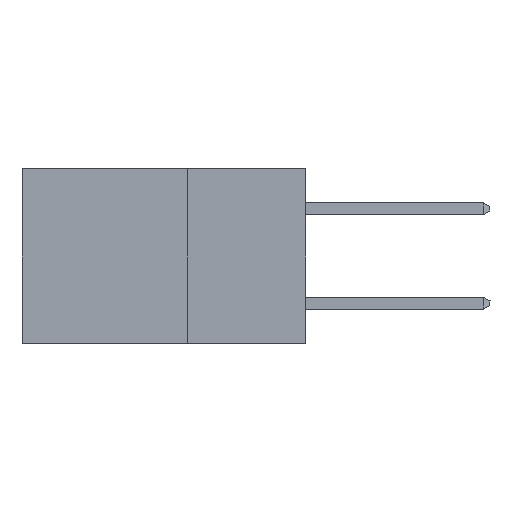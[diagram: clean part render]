
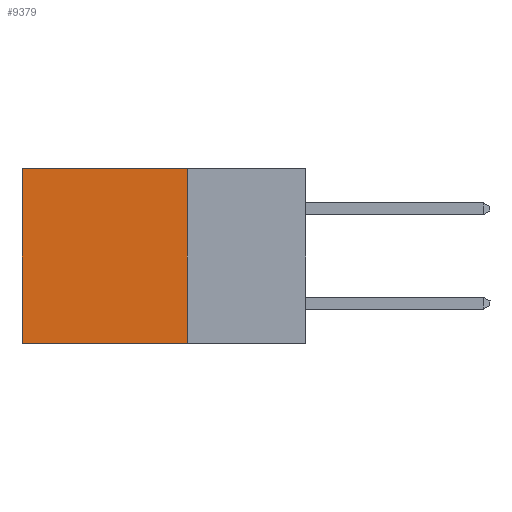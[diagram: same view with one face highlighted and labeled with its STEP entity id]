
A CAD part, left-side view. The second image highlights one B-rep face of the part: STEP entity #9379.
In plain terms, the highlighted planar face has unit normal (-1, 0, 0).
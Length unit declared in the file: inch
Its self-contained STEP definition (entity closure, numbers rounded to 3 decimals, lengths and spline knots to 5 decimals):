
#405 = PLANE ( 'NONE',  #13669 ) ;
#949 = EDGE_LOOP ( 'NONE', ( #6802, #19636, #22752, #12591 ) ) ;
#1035 = EDGE_CURVE ( 'NONE', #9798, #18893, #12178, .T. ) ;
#1588 = LINE ( 'NONE', #6658, #21411 ) ;
#1845 = VECTOR ( 'NONE', #4950, 39.37008 ) ;
#3019 = CARTESIAN_POINT ( 'NONE',  ( 0.2615, 0.25, -0.37 ) ) ;
#4057 = DIRECTION ( 'NONE',  ( 1., 0., 0. ) ) ;
#4217 = VECTOR ( 'NONE', #15095, 39.37008 ) ;
#4950 = DIRECTION ( 'NONE',  ( 0., 1., 0. ) ) ;
#5088 = VERTEX_POINT ( 'NONE', #15208 ) ;
#5269 = VECTOR ( 'NONE', #11151, 39.37008 ) ;
#6658 = CARTESIAN_POINT ( 'NONE',  ( 0.2615, 0.6, -0.37 ) ) ;
#6802 = ORIENTED_EDGE ( 'NONE', *, *, #23432, .T. ) ;
#8105 = CARTESIAN_POINT ( 'NONE',  ( 0.2615, 0.6, -0.37 ) ) ;
#8531 = LINE ( 'NONE', #14786, #5269 ) ;
#9379 = ADVANCED_FACE ( 'NONE', ( #21904 ), #405, .F. ) ;
#9798 = VERTEX_POINT ( 'NONE', #12338 ) ;
#11151 = DIRECTION ( 'NONE',  ( 0., 1., 0. ) ) ;
#11476 = CARTESIAN_POINT ( 'NONE',  ( 0.2615, 0.25, -0.37 ) ) ;
#12178 = LINE ( 'NONE', #3019, #1845 ) ;
#12338 = CARTESIAN_POINT ( 'NONE',  ( 0.2615, 0.25, -0.37 ) ) ;
#12591 = ORIENTED_EDGE ( 'NONE', *, *, #18659, .T. ) ;
#13432 = LINE ( 'NONE', #11476, #4217 ) ;
#13538 = CARTESIAN_POINT ( 'NONE',  ( 0.2615, 0.25, 0. ) ) ;
#13669 = AXIS2_PLACEMENT_3D ( 'NONE', #15021, #4057, #16784 ) ;
#14020 = EDGE_CURVE ( 'NONE', #21846, #9798, #13432, .T. ) ;
#14786 = CARTESIAN_POINT ( 'NONE',  ( 0.2615, 0.25, 0. ) ) ;
#15021 = CARTESIAN_POINT ( 'NONE',  ( 0.2615, 0.25, -0.37 ) ) ;
#15095 = DIRECTION ( 'NONE',  ( 0., 0., -1. ) ) ;
#15208 = CARTESIAN_POINT ( 'NONE',  ( 0.2615, 0.6, 0. ) ) ;
#16784 = DIRECTION ( 'NONE',  ( 0., 0., -1. ) ) ;
#17503 = DIRECTION ( 'NONE',  ( 0., 0., -1. ) ) ;
#18659 = EDGE_CURVE ( 'NONE', #21846, #5088, #8531, .T. ) ;
#18893 = VERTEX_POINT ( 'NONE', #8105 ) ;
#19636 = ORIENTED_EDGE ( 'NONE', *, *, #1035, .F. ) ;
#21411 = VECTOR ( 'NONE', #17503, 39.37008 ) ;
#21846 = VERTEX_POINT ( 'NONE', #13538 ) ;
#21904 = FACE_OUTER_BOUND ( 'NONE', #949, .T. ) ;
#22752 = ORIENTED_EDGE ( 'NONE', *, *, #14020, .F. ) ;
#23432 = EDGE_CURVE ( 'NONE', #5088, #18893, #1588, .T. ) ;
